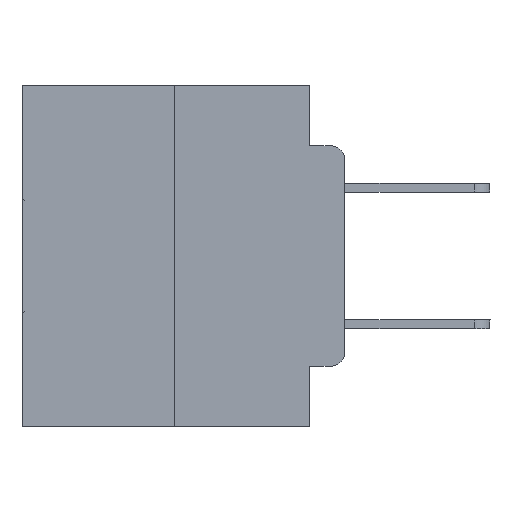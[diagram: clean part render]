
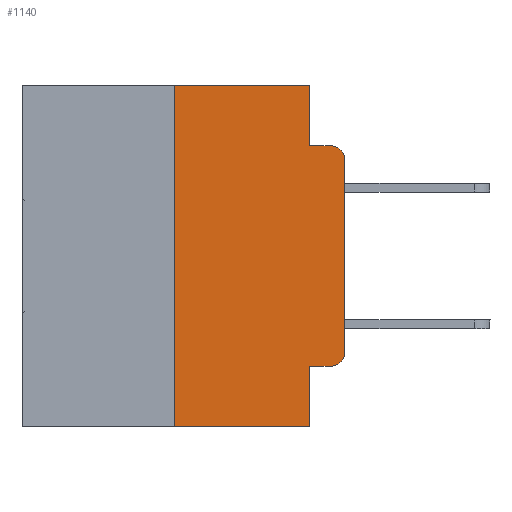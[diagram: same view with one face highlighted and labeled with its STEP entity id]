
A CAD part, left-side view. The second image highlights one B-rep face of the part: STEP entity #1140.
In plain terms, the highlighted planar face has unit normal (-1, 0, 0).
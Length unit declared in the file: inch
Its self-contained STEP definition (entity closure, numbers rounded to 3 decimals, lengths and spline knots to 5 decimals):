
#201 = VECTOR ( 'NONE', #13338, 39.37008 ) ;
#801 = EDGE_CURVE ( 'NONE', #6766, #6357, #17842, .T. ) ;
#1140 = ADVANCED_FACE ( 'NONE', ( #16949 ), #17772, .F. ) ;
#1253 = CARTESIAN_POINT ( 'NONE',  ( 0., 0., -0.3915 ) ) ;
#1367 = VECTOR ( 'NONE', #20346, 39.37008 ) ;
#1369 = CARTESIAN_POINT ( 'NONE',  ( 0., 0.25, 0. ) ) ;
#2267 = CARTESIAN_POINT ( 'NONE',  ( 0., 0.02, -0.0885 ) ) ;
#2282 = CARTESIAN_POINT ( 'NONE',  ( 0., 0.051, -0.0885 ) ) ;
#2385 = CARTESIAN_POINT ( 'NONE',  ( 0., 0., 0. ) ) ;
#2628 = VERTEX_POINT ( 'NONE', #17485 ) ;
#2873 = CARTESIAN_POINT ( 'NONE',  ( 0., 0.02, -0.4115 ) ) ;
#3370 = CARTESIAN_POINT ( 'NONE',  ( 0., 0.02, -0.1085 ) ) ;
#3480 = ORIENTED_EDGE ( 'NONE', *, *, #23472, .F. ) ;
#3503 = EDGE_CURVE ( 'NONE', #14542, #26581, #7873, .T. ) ;
#3636 = ORIENTED_EDGE ( 'NONE', *, *, #3503, .T. ) ;
#3653 = CARTESIAN_POINT ( 'NONE',  ( 0., 0.473, 0. ) ) ;
#3892 = LINE ( 'NONE', #6347, #10137 ) ;
#5247 = LINE ( 'NONE', #21042, #15898 ) ;
#5991 = EDGE_LOOP ( 'NONE', ( #24019, #13138, #11387, #15369, #25515, #21485, #7024, #3480, #12703, #3636 ) ) ;
#6347 = CARTESIAN_POINT ( 'NONE',  ( 0., 0.051, 0. ) ) ;
#6357 = VERTEX_POINT ( 'NONE', #22830 ) ;
#6423 = CARTESIAN_POINT ( 'NONE',  ( 0., 0.02, -0.3915 ) ) ;
#6443 = CARTESIAN_POINT ( 'NONE',  ( 0., 0.051, -0.4115 ) ) ;
#6471 = LINE ( 'NONE', #2385, #201 ) ;
#6766 = VERTEX_POINT ( 'NONE', #22795 ) ;
#7024 = ORIENTED_EDGE ( 'NONE', *, *, #801, .T. ) ;
#7351 = EDGE_CURVE ( 'NONE', #6766, #24919, #23183, .T. ) ;
#7611 = EDGE_CURVE ( 'NONE', #26581, #25464, #6471, .T. ) ;
#7873 = CIRCLE ( 'NONE', #28014, 0.02 ) ;
#7894 = DIRECTION ( 'NONE',  ( 1., 0., 0. ) ) ;
#8124 = DIRECTION ( 'NONE',  ( 0., 0., -1. ) ) ;
#8490 = DIRECTION ( 'NONE',  ( 0., 0., -1. ) ) ;
#9357 = DIRECTION ( 'NONE',  ( 0., -1., 0. ) ) ;
#10137 = VECTOR ( 'NONE', #8124, 39.37008 ) ;
#10830 = DIRECTION ( 'NONE',  ( 0., 0., -1. ) ) ;
#11387 = ORIENTED_EDGE ( 'NONE', *, *, #19157, .F. ) ;
#11422 = CARTESIAN_POINT ( 'NONE',  ( 0., 0.473, -0.5 ) ) ;
#11888 = VECTOR ( 'NONE', #23334, 39.37008 ) ;
#12051 = VECTOR ( 'NONE', #8490, 39.37008 ) ;
#12056 = CARTESIAN_POINT ( 'NONE',  ( 0., 0.25, 0. ) ) ;
#12268 = VECTOR ( 'NONE', #24679, 39.37008 ) ;
#12286 = DIRECTION ( 'NONE',  ( -1., 0., 0. ) ) ;
#12593 = AXIS2_PLACEMENT_3D ( 'NONE', #3653, #7894, #28754 ) ;
#12703 = ORIENTED_EDGE ( 'NONE', *, *, #18741, .T. ) ;
#13030 = LINE ( 'NONE', #6443, #14134 ) ;
#13138 = ORIENTED_EDGE ( 'NONE', *, *, #20315, .T. ) ;
#13338 = DIRECTION ( 'NONE',  ( 0., 0., 1. ) ) ;
#14076 = CARTESIAN_POINT ( 'NONE',  ( 0., 0., -0.1085 ) ) ;
#14134 = VECTOR ( 'NONE', #28685, 39.37008 ) ;
#14542 = VERTEX_POINT ( 'NONE', #2873 ) ;
#15369 = ORIENTED_EDGE ( 'NONE', *, *, #24207, .F. ) ;
#15382 = EDGE_CURVE ( 'NONE', #24919, #22526, #5247, .T. ) ;
#15898 = VECTOR ( 'NONE', #9357, 39.37008 ) ;
#16949 = FACE_OUTER_BOUND ( 'NONE', #5991, .T. ) ;
#17485 = CARTESIAN_POINT ( 'NONE',  ( 0., 0.051, -0.4115 ) ) ;
#17522 = DIRECTION ( 'NONE',  ( -1., 0., 0. ) ) ;
#17772 = PLANE ( 'NONE',  #12593 ) ;
#17842 = LINE ( 'NONE', #11422, #1367 ) ;
#18741 = EDGE_CURVE ( 'NONE', #2628, #14542, #13030, .T. ) ;
#19017 = VERTEX_POINT ( 'NONE', #23557 ) ;
#19157 = EDGE_CURVE ( 'NONE', #19017, #26760, #24960, .T. ) ;
#20315 = EDGE_CURVE ( 'NONE', #25464, #26760, #27793, .T. ) ;
#20346 = DIRECTION ( 'NONE',  ( 0., -1., 0. ) ) ;
#21042 = CARTESIAN_POINT ( 'NONE',  ( 0., 0.473, 0. ) ) ;
#21215 = DIRECTION ( 'NONE',  ( 0., 0., -1. ) ) ;
#21485 = ORIENTED_EDGE ( 'NONE', *, *, #7351, .F. ) ;
#22526 = VERTEX_POINT ( 'NONE', #28514 ) ;
#22795 = CARTESIAN_POINT ( 'NONE',  ( 0., 0.25, -0.5 ) ) ;
#22830 = CARTESIAN_POINT ( 'NONE',  ( 0., 0.051, -0.5 ) ) ;
#23183 = LINE ( 'NONE', #12056, #11888 ) ;
#23334 = DIRECTION ( 'NONE',  ( 0., 0., 1. ) ) ;
#23472 = EDGE_CURVE ( 'NONE', #2628, #6357, #3892, .T. ) ;
#23557 = CARTESIAN_POINT ( 'NONE',  ( 0., 0.051, -0.0885 ) ) ;
#23719 = LINE ( 'NONE', #28221, #12051 ) ;
#24019 = ORIENTED_EDGE ( 'NONE', *, *, #7611, .T. ) ;
#24207 = EDGE_CURVE ( 'NONE', #22526, #19017, #23719, .T. ) ;
#24679 = DIRECTION ( 'NONE',  ( 0., -1., 0. ) ) ;
#24919 = VERTEX_POINT ( 'NONE', #1369 ) ;
#24960 = LINE ( 'NONE', #2282, #12268 ) ;
#25464 = VERTEX_POINT ( 'NONE', #14076 ) ;
#25473 = AXIS2_PLACEMENT_3D ( 'NONE', #3370, #12286, #21215 ) ;
#25515 = ORIENTED_EDGE ( 'NONE', *, *, #15382, .F. ) ;
#26581 = VERTEX_POINT ( 'NONE', #1253 ) ;
#26760 = VERTEX_POINT ( 'NONE', #2267 ) ;
#27793 = CIRCLE ( 'NONE', #25473, 0.02 ) ;
#28014 = AXIS2_PLACEMENT_3D ( 'NONE', #6423, #17522, #10830 ) ;
#28221 = CARTESIAN_POINT ( 'NONE',  ( 0., 0.051, 0. ) ) ;
#28514 = CARTESIAN_POINT ( 'NONE',  ( 0., 0.051, 0. ) ) ;
#28685 = DIRECTION ( 'NONE',  ( 0., -1., 0. ) ) ;
#28754 = DIRECTION ( 'NONE',  ( 0., 0., -1. ) ) ;
